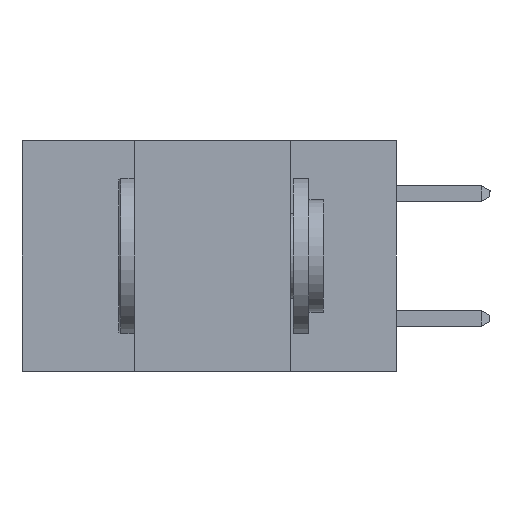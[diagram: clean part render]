
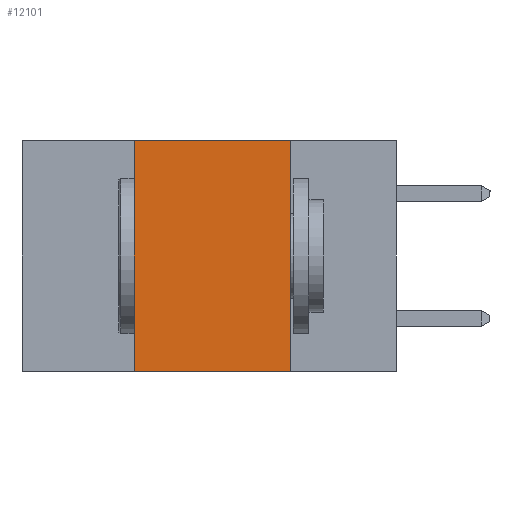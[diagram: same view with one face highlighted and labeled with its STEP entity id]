
A CAD part, left-side view. The second image highlights one B-rep face of the part: STEP entity #12101.
In plain terms, the highlighted planar face has unit normal (-1, 0, 0).
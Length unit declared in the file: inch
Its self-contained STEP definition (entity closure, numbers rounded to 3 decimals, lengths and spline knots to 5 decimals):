
#851 = LINE ( 'NONE', #12383, #9200 ) ;
#1654 = DIRECTION ( 'NONE',  ( 0., 0., 1. ) ) ;
#2780 = EDGE_CURVE ( 'NONE', #17725, #6908, #10341, .T. ) ;
#2889 = DIRECTION ( 'NONE',  ( 0., -1., 0. ) ) ;
#3091 = LINE ( 'NONE', #14584, #5439 ) ;
#3357 = CARTESIAN_POINT ( 'NONE',  ( 0., 0.6, 0. ) ) ;
#3458 = FACE_OUTER_BOUND ( 'NONE', #12838, .T. ) ;
#5439 = VECTOR ( 'NONE', #1654, 39.37008 ) ;
#5463 = LINE ( 'NONE', #6988, #6990 ) ;
#6210 = CARTESIAN_POINT ( 'NONE',  ( 0., 0.42, -0.37 ) ) ;
#6895 = DIRECTION ( 'NONE',  ( 0., 0., -1. ) ) ;
#6908 = VERTEX_POINT ( 'NONE', #17301 ) ;
#6988 = CARTESIAN_POINT ( 'NONE',  ( 0., 0.17, -0.37 ) ) ;
#6990 = VECTOR ( 'NONE', #6895, 39.37008 ) ;
#7245 = EDGE_CURVE ( 'NONE', #16300, #8513, #851, .T. ) ;
#8513 = VERTEX_POINT ( 'NONE', #11661 ) ;
#9033 = CARTESIAN_POINT ( 'NONE',  ( 0., 0.42, 0. ) ) ;
#9200 = VECTOR ( 'NONE', #11166, 39.37008 ) ;
#9213 = PLANE ( 'NONE',  #17425 ) ;
#10239 = CARTESIAN_POINT ( 'NONE',  ( 0., 0.6, 0. ) ) ;
#10341 = LINE ( 'NONE', #10239, #11638 ) ;
#11166 = DIRECTION ( 'NONE',  ( 0., -1., 0. ) ) ;
#11638 = VECTOR ( 'NONE', #2889, 39.37008 ) ;
#11661 = CARTESIAN_POINT ( 'NONE',  ( 0., 0.17, -0.37 ) ) ;
#12101 = ADVANCED_FACE ( 'NONE', ( #3458 ), #9213, .F. ) ;
#12383 = CARTESIAN_POINT ( 'NONE',  ( 0., 0.6, -0.37 ) ) ;
#12838 = EDGE_LOOP ( 'NONE', ( #18489, #16432, #15318, #14989 ) ) ;
#13347 = DIRECTION ( 'NONE',  ( 1., 0., 0. ) ) ;
#13472 = EDGE_CURVE ( 'NONE', #16300, #17725, #3091, .T. ) ;
#14407 = EDGE_CURVE ( 'NONE', #6908, #8513, #5463, .T. ) ;
#14584 = CARTESIAN_POINT ( 'NONE',  ( 0., 0.42, -0.37 ) ) ;
#14989 = ORIENTED_EDGE ( 'NONE', *, *, #7245, .T. ) ;
#15318 = ORIENTED_EDGE ( 'NONE', *, *, #13472, .F. ) ;
#16300 = VERTEX_POINT ( 'NONE', #6210 ) ;
#16432 = ORIENTED_EDGE ( 'NONE', *, *, #2780, .F. ) ;
#17301 = CARTESIAN_POINT ( 'NONE',  ( 0., 0.17, 0. ) ) ;
#17425 = AXIS2_PLACEMENT_3D ( 'NONE', #3357, #13347, #17755 ) ;
#17725 = VERTEX_POINT ( 'NONE', #9033 ) ;
#17755 = DIRECTION ( 'NONE',  ( 0., 0., -1. ) ) ;
#18489 = ORIENTED_EDGE ( 'NONE', *, *, #14407, .F. ) ;
